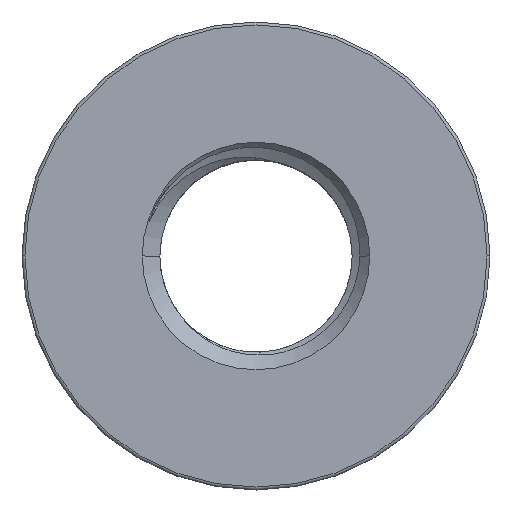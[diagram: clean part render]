
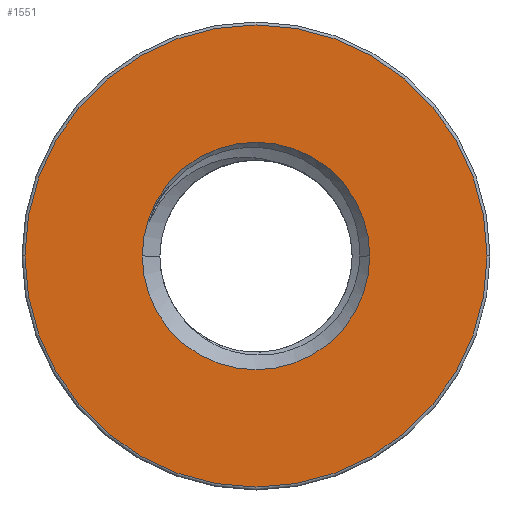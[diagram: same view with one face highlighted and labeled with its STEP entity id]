
A CAD part, top view. The second image highlights one B-rep face of the part: STEP entity #1551.
In plain terms, the highlighted planar face has unit normal (0, 0, 1).
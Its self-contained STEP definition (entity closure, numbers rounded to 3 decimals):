
#13 = CARTESIAN_POINT ( 'NONE',  ( 0., 0., 0. ) ) ;
#31 = DIRECTION ( 'NONE',  ( 0., 0., 1. ) ) ;
#115 = CIRCLE ( 'NONE', #623, 3.918 ) ;
#128 = DIRECTION ( 'NONE',  ( -1., 0., 0. ) ) ;
#184 = DIRECTION ( 'NONE',  ( -1., 0., 0. ) ) ;
#219 = EDGE_LOOP ( 'NONE', ( #335, #366 ) ) ;
#228 = CIRCLE ( 'NONE', #689, 1.929 ) ;
#273 = CIRCLE ( 'NONE', #669, 3.918 ) ;
#335 = ORIENTED_EDGE ( 'NONE', *, *, #1796, .T. ) ;
#366 = ORIENTED_EDGE ( 'NONE', *, *, #1509, .T. ) ;
#435 = AXIS2_PLACEMENT_3D ( 'NONE', #13, #1192, #184 ) ;
#439 = CARTESIAN_POINT ( 'NONE',  ( 1.929, 0., 0. ) ) ;
#472 = DIRECTION ( 'NONE',  ( 0., 0., 1. ) ) ;
#614 = AXIS2_PLACEMENT_3D ( 'NONE', #655, #833, #2056 ) ;
#623 = AXIS2_PLACEMENT_3D ( 'NONE', #1038, #31, #1209 ) ;
#655 = CARTESIAN_POINT ( 'NONE',  ( 0., 1.629, 0. ) ) ;
#669 = AXIS2_PLACEMENT_3D ( 'NONE', #1495, #472, #1681 ) ;
#689 = AXIS2_PLACEMENT_3D ( 'NONE', #2189, #1137, #128 ) ;
#749 = ORIENTED_EDGE ( 'NONE', *, *, #1515, .T. ) ;
#810 = VERTEX_POINT ( 'NONE', #439 ) ;
#833 = DIRECTION ( 'NONE',  ( 0., 0., -1. ) ) ;
#1011 = FACE_BOUND ( 'NONE', #219, .T. ) ;
#1038 = CARTESIAN_POINT ( 'NONE',  ( 0., 0., 0. ) ) ;
#1137 = DIRECTION ( 'NONE',  ( 0., 0., -1. ) ) ;
#1192 = DIRECTION ( 'NONE',  ( 0., 0., -1. ) ) ;
#1209 = DIRECTION ( 'NONE',  ( 1., 0., 0. ) ) ;
#1458 = EDGE_LOOP ( 'NONE', ( #1693, #749 ) ) ;
#1495 = CARTESIAN_POINT ( 'NONE',  ( 0., 0., 0. ) ) ;
#1509 = EDGE_CURVE ( 'NONE', #1791, #810, #228, .T. ) ;
#1515 = EDGE_CURVE ( 'NONE', #1708, #1854, #273, .T. ) ;
#1551 = ADVANCED_FACE ( 'NONE', ( #1011, #1975 ), #2051, .F. ) ;
#1575 = EDGE_CURVE ( 'NONE', #1854, #1708, #115, .T. ) ;
#1681 = DIRECTION ( 'NONE',  ( 1., 0., 0. ) ) ;
#1693 = ORIENTED_EDGE ( 'NONE', *, *, #1575, .T. ) ;
#1708 = VERTEX_POINT ( 'NONE', #2201 ) ;
#1791 = VERTEX_POINT ( 'NONE', #1917 ) ;
#1796 = EDGE_CURVE ( 'NONE', #810, #1791, #1952, .T. ) ;
#1854 = VERTEX_POINT ( 'NONE', #2106 ) ;
#1917 = CARTESIAN_POINT ( 'NONE',  ( -1.929, 0., 0. ) ) ;
#1952 = CIRCLE ( 'NONE', #435, 1.929 ) ;
#1975 = FACE_OUTER_BOUND ( 'NONE', #1458, .T. ) ;
#2051 = PLANE ( 'NONE',  #614 ) ;
#2056 = DIRECTION ( 'NONE',  ( -1., 0., 0. ) ) ;
#2106 = CARTESIAN_POINT ( 'NONE',  ( 3.918, 0., 0. ) ) ;
#2189 = CARTESIAN_POINT ( 'NONE',  ( 0., 0., 0. ) ) ;
#2201 = CARTESIAN_POINT ( 'NONE',  ( -3.918, 0., 0. ) ) ;
